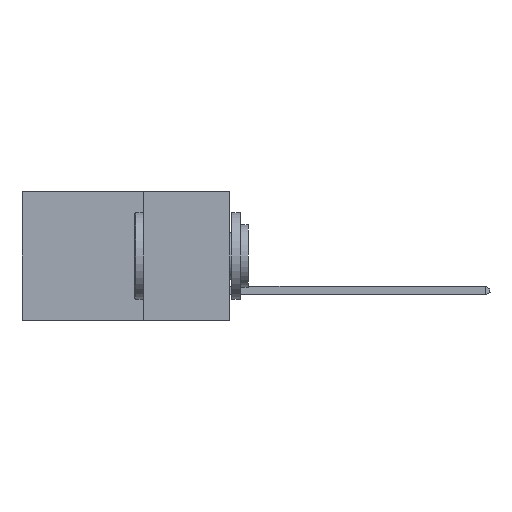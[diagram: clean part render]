
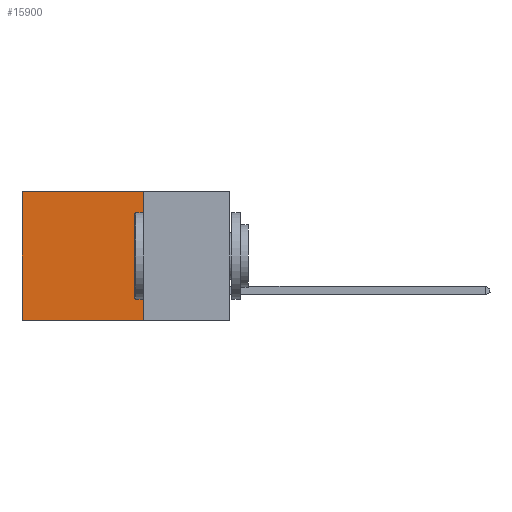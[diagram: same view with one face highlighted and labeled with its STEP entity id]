
A CAD part, left-side view. The second image highlights one B-rep face of the part: STEP entity #15900.
In plain terms, the highlighted planar face has unit normal (-1, 0, 0).
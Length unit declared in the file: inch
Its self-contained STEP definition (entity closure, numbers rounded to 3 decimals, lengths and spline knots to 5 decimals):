
#72 = VECTOR ( 'NONE', #4134, 39.37008 ) ;
#662 = ORIENTED_EDGE ( 'NONE', *, *, #10598, .F. ) ;
#691 = CARTESIAN_POINT ( 'NONE',  ( 0.298, 0.25, 0. ) ) ;
#1506 = CARTESIAN_POINT ( 'NONE',  ( 0.298, 0.25, 0. ) ) ;
#1701 = VECTOR ( 'NONE', #9623, 39.37008 ) ;
#1821 = FACE_OUTER_BOUND ( 'NONE', #12478, .T. ) ;
#2915 = DIRECTION ( 'NONE',  ( 1., 0., 0. ) ) ;
#3442 = VERTEX_POINT ( 'NONE', #9267 ) ;
#3479 = VERTEX_POINT ( 'NONE', #7980 ) ;
#4057 = LINE ( 'NONE', #691, #14379 ) ;
#4134 = DIRECTION ( 'NONE',  ( 0., 1., 0. ) ) ;
#4546 = ORIENTED_EDGE ( 'NONE', *, *, #13145, .T. ) ;
#5719 = DIRECTION ( 'NONE',  ( 0., 0., -1. ) ) ;
#6212 = EDGE_CURVE ( 'NONE', #14961, #3479, #6492, .T. ) ;
#6492 = LINE ( 'NONE', #16626, #1701 ) ;
#6937 = PLANE ( 'NONE',  #10562 ) ;
#7740 = CARTESIAN_POINT ( 'NONE',  ( 0.298, 0.6, -0.37 ) ) ;
#7980 = CARTESIAN_POINT ( 'NONE',  ( 0.298, 0.25, -0.37 ) ) ;
#8294 = CARTESIAN_POINT ( 'NONE',  ( 0.298, 0.6, 0. ) ) ;
#9011 = ORIENTED_EDGE ( 'NONE', *, *, #6212, .F. ) ;
#9267 = CARTESIAN_POINT ( 'NONE',  ( 0.298, 0.6, 0. ) ) ;
#9566 = CARTESIAN_POINT ( 'NONE',  ( 0.298, 0.25, -0.37 ) ) ;
#9623 = DIRECTION ( 'NONE',  ( 0., 0., -1. ) ) ;
#9881 = CARTESIAN_POINT ( 'NONE',  ( 0.298, 0.25, 0. ) ) ;
#9963 = DIRECTION ( 'NONE',  ( 0., 0., -1. ) ) ;
#10468 = DIRECTION ( 'NONE',  ( 0., 1., 0. ) ) ;
#10562 = AXIS2_PLACEMENT_3D ( 'NONE', #1506, #2915, #5719 ) ;
#10598 = EDGE_CURVE ( 'NONE', #3479, #11466, #15442, .T. ) ;
#11149 = LINE ( 'NONE', #8294, #15552 ) ;
#11466 = VERTEX_POINT ( 'NONE', #7740 ) ;
#11896 = ORIENTED_EDGE ( 'NONE', *, *, #15439, .T. ) ;
#12478 = EDGE_LOOP ( 'NONE', ( #4546, #662, #9011, #11896 ) ) ;
#13145 = EDGE_CURVE ( 'NONE', #3442, #11466, #11149, .T. ) ;
#14379 = VECTOR ( 'NONE', #10468, 39.37008 ) ;
#14961 = VERTEX_POINT ( 'NONE', #9881 ) ;
#15439 = EDGE_CURVE ( 'NONE', #14961, #3442, #4057, .T. ) ;
#15442 = LINE ( 'NONE', #9566, #72 ) ;
#15552 = VECTOR ( 'NONE', #9963, 39.37008 ) ;
#15900 = ADVANCED_FACE ( 'NONE', ( #1821 ), #6937, .F. ) ;
#16626 = CARTESIAN_POINT ( 'NONE',  ( 0.298, 0.25, 0. ) ) ;
